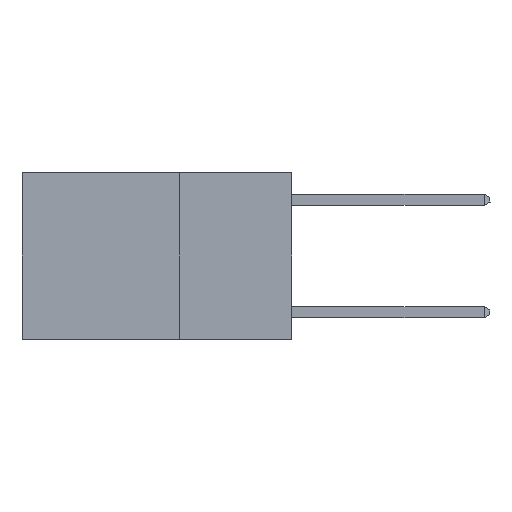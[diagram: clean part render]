
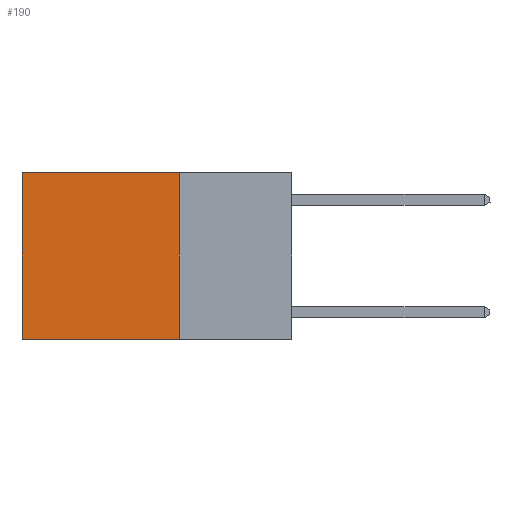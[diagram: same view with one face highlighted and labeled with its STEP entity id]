
A CAD part, left-side view. The second image highlights one B-rep face of the part: STEP entity #190.
In plain terms, the highlighted planar face has unit normal (-1, 0, 0).
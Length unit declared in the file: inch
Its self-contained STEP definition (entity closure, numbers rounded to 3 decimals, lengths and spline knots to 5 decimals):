
#190 = ADVANCED_FACE ( 'NONE', ( #16508 ), #3299, .F. ) ;
#888 = VECTOR ( 'NONE', #13430, 39.37008 ) ;
#1671 = EDGE_CURVE ( 'NONE', #16832, #8544, #8358, .T. ) ;
#2354 = VECTOR ( 'NONE', #10299, 39.37008 ) ;
#3299 = PLANE ( 'NONE',  #13820 ) ;
#4729 = DIRECTION ( 'NONE',  ( 0., 0., -1. ) ) ;
#4834 = CARTESIAN_POINT ( 'NONE',  ( 0.2625, 0.25, 0. ) ) ;
#5479 = ORIENTED_EDGE ( 'NONE', *, *, #1671, .T. ) ;
#5953 = VERTEX_POINT ( 'NONE', #6949 ) ;
#6064 = DIRECTION ( 'NONE',  ( 0., 0., -1. ) ) ;
#6590 = ORIENTED_EDGE ( 'NONE', *, *, #16414, .F. ) ;
#6949 = CARTESIAN_POINT ( 'NONE',  ( 0.2625, 0.25, 0. ) ) ;
#7131 = LINE ( 'NONE', #4834, #8580 ) ;
#7307 = DIRECTION ( 'NONE',  ( 0., 0., -1. ) ) ;
#7603 = CARTESIAN_POINT ( 'NONE',  ( 0.2625, 0.25, -0.37 ) ) ;
#7984 = CARTESIAN_POINT ( 'NONE',  ( 0.2625, 0.6, -0.37 ) ) ;
#8358 = LINE ( 'NONE', #15404, #16432 ) ;
#8428 = EDGE_CURVE ( 'NONE', #5953, #16832, #11399, .T. ) ;
#8544 = VERTEX_POINT ( 'NONE', #7984 ) ;
#8580 = VECTOR ( 'NONE', #6064, 39.37008 ) ;
#8757 = CARTESIAN_POINT ( 'NONE',  ( 0.2625, 0.25, 0. ) ) ;
#8799 = VERTEX_POINT ( 'NONE', #15151 ) ;
#10299 = DIRECTION ( 'NONE',  ( 0., 1., 0. ) ) ;
#11399 = LINE ( 'NONE', #14573, #888 ) ;
#11833 = EDGE_CURVE ( 'NONE', #8799, #8544, #12442, .T. ) ;
#12442 = LINE ( 'NONE', #7603, #2354 ) ;
#13430 = DIRECTION ( 'NONE',  ( 0., 1., 0. ) ) ;
#13478 = CARTESIAN_POINT ( 'NONE',  ( 0.2625, 0.6, 0. ) ) ;
#13712 = ORIENTED_EDGE ( 'NONE', *, *, #11833, .F. ) ;
#13820 = AXIS2_PLACEMENT_3D ( 'NONE', #8757, #16451, #7307 ) ;
#14049 = EDGE_LOOP ( 'NONE', ( #5479, #13712, #6590, #15102 ) ) ;
#14573 = CARTESIAN_POINT ( 'NONE',  ( 0.2625, 0.25, 0. ) ) ;
#15102 = ORIENTED_EDGE ( 'NONE', *, *, #8428, .T. ) ;
#15151 = CARTESIAN_POINT ( 'NONE',  ( 0.2625, 0.25, -0.37 ) ) ;
#15404 = CARTESIAN_POINT ( 'NONE',  ( 0.2625, 0.6, 0. ) ) ;
#16414 = EDGE_CURVE ( 'NONE', #5953, #8799, #7131, .T. ) ;
#16432 = VECTOR ( 'NONE', #4729, 39.37008 ) ;
#16451 = DIRECTION ( 'NONE',  ( 1., 0., 0. ) ) ;
#16508 = FACE_OUTER_BOUND ( 'NONE', #14049, .T. ) ;
#16832 = VERTEX_POINT ( 'NONE', #13478 ) ;
